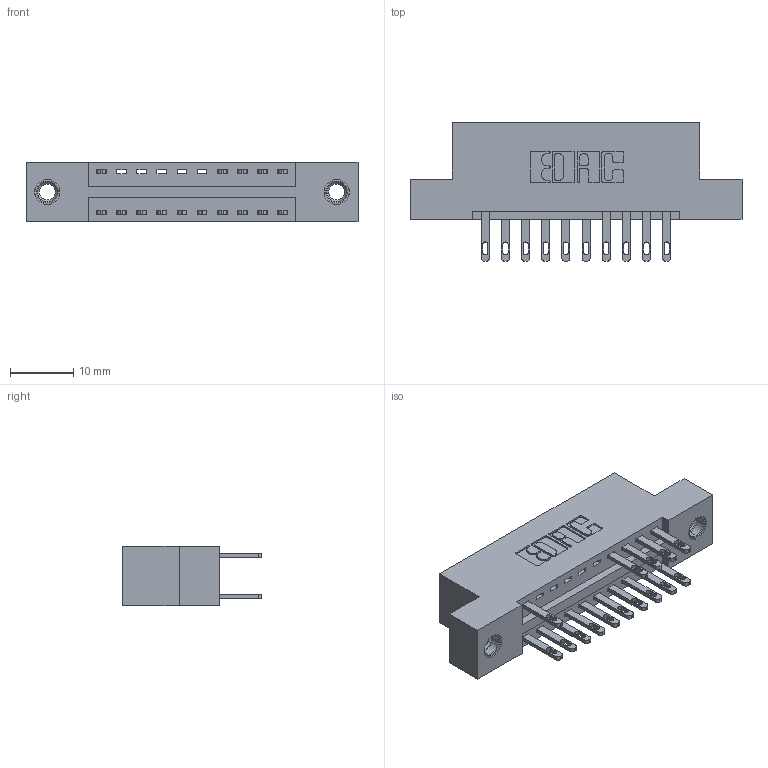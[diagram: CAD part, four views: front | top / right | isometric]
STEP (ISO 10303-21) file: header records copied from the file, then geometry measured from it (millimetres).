
FILE_DESCRIPTION (( 'STEP AP203' ), '1' );
FILE_NAME ('346-020-500-207.STEP', '2018-08-20T10:46:09', ( '' ), ( '' ), 'SwSTEP 2.0', 'SolidWorks 2016', '' );
FILE_SCHEMA (( 'CONFIG_CONTROL_DESIGN' ));
Length unit declared in the file: inch
Products named in the file (4): 346 Part_Flush Mounting Lugs - 0.156 Dia-TI; 345-292-001_345-293-100; 345-250-001_345-250-005-103; 346-020-500-207
Assembly tree (18 placements, depth 2):
  346-020-500-207
    346 Part_Flush Mounting Lugs - 0.156 Dia-TI
    345-292-001_345-293-100  x15
    345-250-001_345-250-005-103  x2
Bounding box: 52.32 x 21.84 x 9.4 mm (x, y, z)
Volume: 4841 mm3; surface area: 6082.6 mm2
Topology: 18 solids, 18 shells, 932 faces, 2775 edges, 1842 vertices
Faces by surface type: plane 568, cylinder 348, cone 12, torus 4
Entity records: 11790 total; most frequent: CARTESIAN_POINT 1990, ORIENTED_EDGE 1922, DIRECTION 1829, EDGE_CURVE 961, LINE 765, VECTOR 765, VERTEX_POINT 636, AXIS2_PLACEMENT_3D 532
